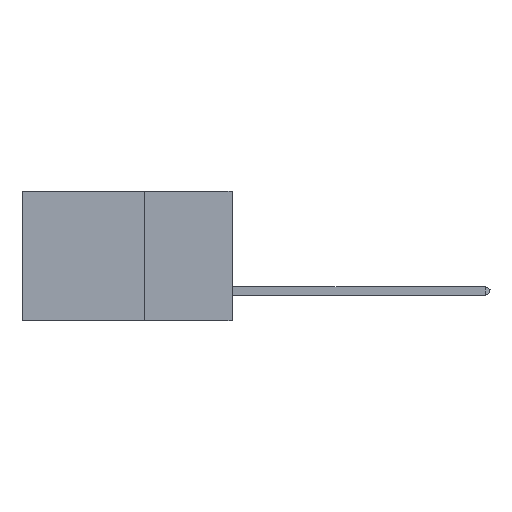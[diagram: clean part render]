
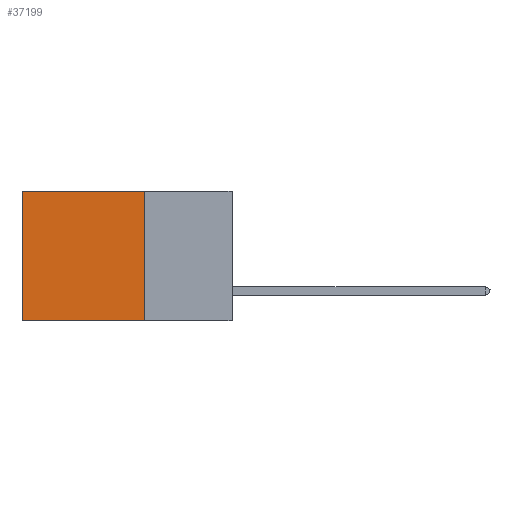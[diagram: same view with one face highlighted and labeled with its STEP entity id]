
A CAD part, left-side view. The second image highlights one B-rep face of the part: STEP entity #37199.
In plain terms, the highlighted planar face has unit normal (-1, 0, 0).
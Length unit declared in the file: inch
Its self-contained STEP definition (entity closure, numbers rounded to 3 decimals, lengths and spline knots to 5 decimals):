
#735 = ORIENTED_EDGE ( 'NONE', *, *, #1304, .T. ) ;
#815 = CARTESIAN_POINT ( 'NONE',  ( 0.2875, 0.6, 0. ) ) ;
#1046 = DIRECTION ( 'NONE',  ( 0., 0., -1. ) ) ;
#1304 = EDGE_CURVE ( 'NONE', #13619, #37405, #28781, .T. ) ;
#3030 = EDGE_LOOP ( 'NONE', ( #735, #34853, #25657, #37886 ) ) ;
#4272 = VECTOR ( 'NONE', #30486, 39.37008 ) ;
#4444 = CARTESIAN_POINT ( 'NONE',  ( 0.2875, 0.6, 0. ) ) ;
#6305 = DIRECTION ( 'NONE',  ( 0., 1., 0. ) ) ;
#7379 = LINE ( 'NONE', #28232, #35349 ) ;
#7676 = AXIS2_PLACEMENT_3D ( 'NONE', #41839, #45685, #1046 ) ;
#7848 = EDGE_CURVE ( 'NONE', #16674, #37405, #35257, .T. ) ;
#11767 = DIRECTION ( 'NONE',  ( 0., 0., -1. ) ) ;
#13619 = VERTEX_POINT ( 'NONE', #4444 ) ;
#13741 = VECTOR ( 'NONE', #11767, 39.37008 ) ;
#14854 = LINE ( 'NONE', #19173, #4272 ) ;
#16340 = VERTEX_POINT ( 'NONE', #42045 ) ;
#16674 = VERTEX_POINT ( 'NONE', #34233 ) ;
#19173 = CARTESIAN_POINT ( 'NONE',  ( 0.2875, 0.25, 0. ) ) ;
#24522 = DIRECTION ( 'NONE',  ( 0., 1., 0. ) ) ;
#25657 = ORIENTED_EDGE ( 'NONE', *, *, #41066, .F. ) ;
#28077 = CARTESIAN_POINT ( 'NONE',  ( 0.2875, 0.25, -0.37 ) ) ;
#28232 = CARTESIAN_POINT ( 'NONE',  ( 0.2875, 0.25, 0. ) ) ;
#28681 = EDGE_CURVE ( 'NONE', #16340, #13619, #7379, .T. ) ;
#28781 = LINE ( 'NONE', #815, #13741 ) ;
#30270 = FACE_OUTER_BOUND ( 'NONE', #3030, .T. ) ;
#30486 = DIRECTION ( 'NONE',  ( 0., 0., -1. ) ) ;
#31148 = VECTOR ( 'NONE', #24522, 39.37008 ) ;
#32470 = CARTESIAN_POINT ( 'NONE',  ( 0.2875, 0.6, -0.37 ) ) ;
#34233 = CARTESIAN_POINT ( 'NONE',  ( 0.2875, 0.25, -0.37 ) ) ;
#34853 = ORIENTED_EDGE ( 'NONE', *, *, #7848, .F. ) ;
#35257 = LINE ( 'NONE', #28077, #31148 ) ;
#35349 = VECTOR ( 'NONE', #6305, 39.37008 ) ;
#37199 = ADVANCED_FACE ( 'NONE', ( #30270 ), #37701, .F. ) ;
#37405 = VERTEX_POINT ( 'NONE', #32470 ) ;
#37701 = PLANE ( 'NONE',  #7676 ) ;
#37886 = ORIENTED_EDGE ( 'NONE', *, *, #28681, .T. ) ;
#41066 = EDGE_CURVE ( 'NONE', #16340, #16674, #14854, .T. ) ;
#41839 = CARTESIAN_POINT ( 'NONE',  ( 0.2875, 0.25, 0. ) ) ;
#42045 = CARTESIAN_POINT ( 'NONE',  ( 0.2875, 0.25, 0. ) ) ;
#45685 = DIRECTION ( 'NONE',  ( 1., 0., 0. ) ) ;
